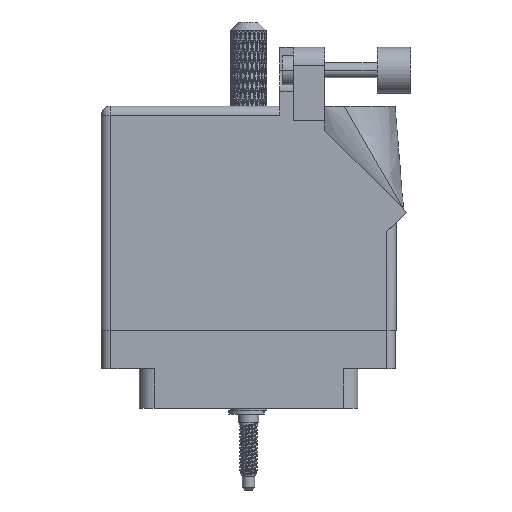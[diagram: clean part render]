
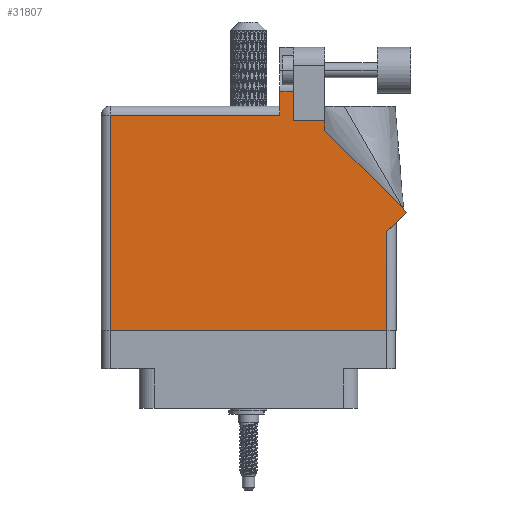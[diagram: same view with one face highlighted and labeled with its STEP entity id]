
A CAD part, front view. The second image highlights one B-rep face of the part: STEP entity #31807.
In plain terms, the highlighted face is planar.
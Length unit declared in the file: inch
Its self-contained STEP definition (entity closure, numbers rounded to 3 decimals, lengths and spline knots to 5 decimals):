
#1335 = DIRECTION ( 'NONE',  ( -1., 0., 0. ) ) ;
#4358 = VECTOR ( 'NONE', #76230, 39.37008 ) ;
#5325 = EDGE_LOOP ( 'NONE', ( #69963, #45018, #97222, #37466, #21062, #10344, #62425, #11141, #54216, #61413, #36127 ) ) ;
#7222 = DIRECTION ( 'NONE',  ( 0.707, 0.707, 0. ) ) ;
#10344 = ORIENTED_EDGE ( 'NONE', *, *, #56427, .T. ) ;
#11141 = ORIENTED_EDGE ( 'NONE', *, *, #72273, .T. ) ;
#16140 = CARTESIAN_POINT ( 'NONE',  ( 0.062, 1.468, 0. ) ) ;
#16179 = VECTOR ( 'NONE', #90884, 39.37008 ) ;
#16330 = VERTEX_POINT ( 'NONE', #62975 ) ;
#18081 = FACE_OUTER_BOUND ( 'NONE', #5325, .T. ) ;
#18325 = DIRECTION ( 'NONE',  ( -1., 0., 0. ) ) ;
#19765 = LINE ( 'NONE', #74857, #103532 ) ;
#21062 = ORIENTED_EDGE ( 'NONE', *, *, #59070, .T. ) ;
#21079 = VERTEX_POINT ( 'NONE', #55459 ) ;
#22345 = EDGE_CURVE ( 'NONE', #68268, #16330, #29947, .T. ) ;
#23332 = CARTESIAN_POINT ( 'NONE',  ( 1.524, 1.43, 0. ) ) ;
#23609 = VECTOR ( 'NONE', #75046, 39.37008 ) ;
#24232 = LINE ( 'NONE', #66860, #48373 ) ;
#25218 = CARTESIAN_POINT ( 'NONE',  ( 1.948, 0.737, 0. ) ) ;
#25491 = CARTESIAN_POINT ( 'NONE',  ( 1.524, 1.43, 0. ) ) ;
#27276 = VECTOR ( 'NONE', #50097, 39.37008 ) ;
#29469 = LINE ( 'NONE', #43277, #53579 ) ;
#29947 = LINE ( 'NONE', #25491, #23609 ) ;
#31807 = ADVANCED_FACE ( 'NONE', ( #18081 ), #88358, .F. ) ;
#32420 = DIRECTION ( 'NONE',  ( -1., 0., 0. ) ) ;
#34405 = CARTESIAN_POINT ( 'NONE',  ( 0., 1.468, 0. ) ) ;
#34863 = DIRECTION ( 'NONE',  ( 0., -1., 0. ) ) ;
#35100 = EDGE_CURVE ( 'NONE', #102439, #44388, #92497, .T. ) ;
#35122 = DIRECTION ( 'NONE',  ( 0., -1., 0. ) ) ;
#35811 = DIRECTION ( 'NONE',  ( 0., 1., 0. ) ) ;
#36127 = ORIENTED_EDGE ( 'NONE', *, *, #22345, .T. ) ;
#37466 = ORIENTED_EDGE ( 'NONE', *, *, #82210, .T. ) ;
#37762 = EDGE_CURVE ( 'NONE', #94784, #21079, #19765, .T. ) ;
#39081 = CARTESIAN_POINT ( 'NONE',  ( 1.524, 1.36442, 0. ) ) ;
#39894 = CARTESIAN_POINT ( 'NONE',  ( 2.01, 0.737, 0. ) ) ;
#40032 = DIRECTION ( 'NONE',  ( 0., 1., 0. ) ) ;
#41870 = CARTESIAN_POINT ( 'NONE',  ( 2.08071, 0.80771, 0. ) ) ;
#43277 = CARTESIAN_POINT ( 'NONE',  ( 0.062, 0., 0. ) ) ;
#43287 = EDGE_CURVE ( 'NONE', #62024, #94784, #24232, .T. ) ;
#43322 = CARTESIAN_POINT ( 'NONE',  ( 1.948, 0., 0. ) ) ;
#44388 = VERTEX_POINT ( 'NONE', #84286 ) ;
#45018 = ORIENTED_EDGE ( 'NONE', *, *, #43287, .T. ) ;
#48373 = VECTOR ( 'NONE', #18325, 39.37008 ) ;
#48980 = VECTOR ( 'NONE', #1335, 39.37008 ) ;
#50097 = DIRECTION ( 'NONE',  ( 0., 1., 0. ) ) ;
#50351 = LINE ( 'NONE', #39894, #82126 ) ;
#51840 = VERTEX_POINT ( 'NONE', #39081 ) ;
#53269 = VERTEX_POINT ( 'NONE', #16140 ) ;
#53427 = EDGE_CURVE ( 'NONE', #53784, #51840, #93533, .T. ) ;
#53579 = VECTOR ( 'NONE', #35122, 39.37008 ) ;
#53784 = VERTEX_POINT ( 'NONE', #41870 ) ;
#54031 = EDGE_CURVE ( 'NONE', #16330, #62024, #90928, .T. ) ;
#54216 = ORIENTED_EDGE ( 'NONE', *, *, #53427, .T. ) ;
#55206 = LINE ( 'NONE', #68072, #4358 ) ;
#55459 = CARTESIAN_POINT ( 'NONE',  ( 1.217, 1.468, 0. ) ) ;
#56427 = EDGE_CURVE ( 'NONE', #77318, #102439, #55206, .T. ) ;
#59070 = EDGE_CURVE ( 'NONE', #53269, #77318, #29469, .T. ) ;
#61413 = ORIENTED_EDGE ( 'NONE', *, *, #82705, .T. ) ;
#62024 = VERTEX_POINT ( 'NONE', #72051 ) ;
#62425 = ORIENTED_EDGE ( 'NONE', *, *, #35100, .T. ) ;
#62975 = CARTESIAN_POINT ( 'NONE',  ( 1.311, 1.43, 0. ) ) ;
#66860 = CARTESIAN_POINT ( 'NONE',  ( 1.64177, 1.6315, 0. ) ) ;
#68072 = CARTESIAN_POINT ( 'NONE',  ( 0., 0., 0. ) ) ;
#68268 = VERTEX_POINT ( 'NONE', #23332 ) ;
#68336 = CARTESIAN_POINT ( 'NONE',  ( 0.062, 0., 0. ) ) ;
#69963 = ORIENTED_EDGE ( 'NONE', *, *, #54031, .T. ) ;
#70878 = VECTOR ( 'NONE', #35811, 39.37008 ) ;
#72051 = CARTESIAN_POINT ( 'NONE',  ( 1.311, 1.6315, 0. ) ) ;
#72273 = EDGE_CURVE ( 'NONE', #44388, #53784, #50351, .T. ) ;
#73754 = CARTESIAN_POINT ( 'NONE',  ( 1.524, 1.36442, 0. ) ) ;
#74857 = CARTESIAN_POINT ( 'NONE',  ( 1.217, 1.53, 0. ) ) ;
#75046 = DIRECTION ( 'NONE',  ( -1., 0., 0. ) ) ;
#76230 = DIRECTION ( 'NONE',  ( 1., 0., 0. ) ) ;
#77318 = VERTEX_POINT ( 'NONE', #68336 ) ;
#80208 = DIRECTION ( 'NONE',  ( 0., 0., -1. ) ) ;
#82126 = VECTOR ( 'NONE', #7222, 39.37008 ) ;
#82210 = EDGE_CURVE ( 'NONE', #21079, #53269, #95822, .T. ) ;
#82697 = CARTESIAN_POINT ( 'NONE',  ( 0., 1.53, 0. ) ) ;
#82705 = EDGE_CURVE ( 'NONE', #51840, #68268, #102181, .T. ) ;
#82771 = AXIS2_PLACEMENT_3D ( 'NONE', #82697, #80208, #32420 ) ;
#84286 = CARTESIAN_POINT ( 'NONE',  ( 1.948, 0.675, 0. ) ) ;
#88358 = PLANE ( 'NONE',  #82771 ) ;
#88378 = VECTOR ( 'NONE', #40032, 39.37008 ) ;
#90884 = DIRECTION ( 'NONE',  ( -0.707, 0.707, 0. ) ) ;
#90928 = LINE ( 'NONE', #103886, #88378 ) ;
#92497 = LINE ( 'NONE', #25218, #70878 ) ;
#93533 = LINE ( 'NONE', #99440, #16179 ) ;
#94784 = VERTEX_POINT ( 'NONE', #100906 ) ;
#95822 = LINE ( 'NONE', #34405, #48980 ) ;
#97222 = ORIENTED_EDGE ( 'NONE', *, *, #37762, .T. ) ;
#99440 = CARTESIAN_POINT ( 'NONE',  ( 2.08071, 0.80771, 0. ) ) ;
#100906 = CARTESIAN_POINT ( 'NONE',  ( 1.217, 1.6315, 0. ) ) ;
#102181 = LINE ( 'NONE', #73754, #27276 ) ;
#102439 = VERTEX_POINT ( 'NONE', #43322 ) ;
#103532 = VECTOR ( 'NONE', #34863, 39.37008 ) ;
#103886 = CARTESIAN_POINT ( 'NONE',  ( 1.311, 1.43, 0. ) ) ;
